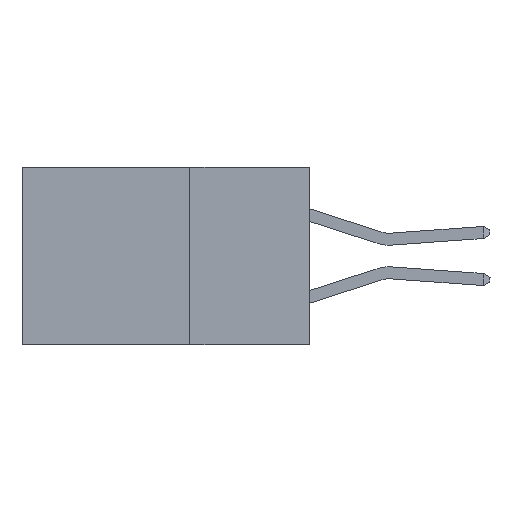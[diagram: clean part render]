
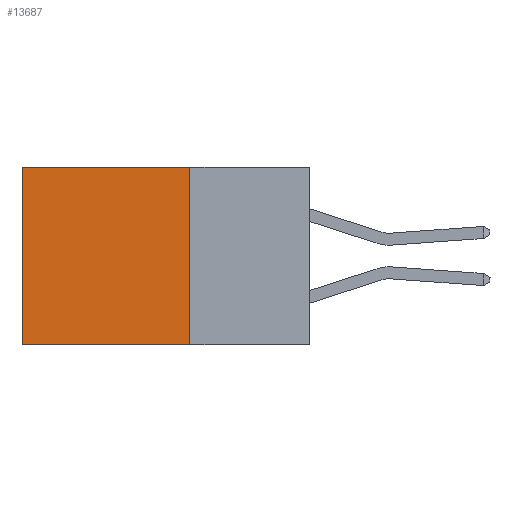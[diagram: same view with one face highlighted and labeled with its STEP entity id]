
A CAD part, left-side view. The second image highlights one B-rep face of the part: STEP entity #13687.
In plain terms, the highlighted planar face has unit normal (-1, 0, 0).
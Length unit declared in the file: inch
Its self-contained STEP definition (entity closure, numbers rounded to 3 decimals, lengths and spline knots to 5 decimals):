
#252 = CARTESIAN_POINT ( 'NONE',  ( 0.2615, 0.25, -0.37 ) ) ;
#585 = LINE ( 'NONE', #252, #17036 ) ;
#797 = CARTESIAN_POINT ( 'NONE',  ( 0.2615, 0.6, -0.37 ) ) ;
#1308 = VERTEX_POINT ( 'NONE', #10513 ) ;
#1394 = DIRECTION ( 'NONE',  ( 0., 0., -1. ) ) ;
#1459 = EDGE_CURVE ( 'NONE', #1308, #5428, #2092, .T. ) ;
#1609 = CARTESIAN_POINT ( 'NONE',  ( 0.2615, 0.6, 0. ) ) ;
#1669 = VERTEX_POINT ( 'NONE', #16102 ) ;
#2092 = LINE ( 'NONE', #4563, #17542 ) ;
#2621 = CARTESIAN_POINT ( 'NONE',  ( 0.2615, 0.25, -0.37 ) ) ;
#2965 = CARTESIAN_POINT ( 'NONE',  ( 0.2615, 0.6, -0.37 ) ) ;
#4163 = DIRECTION ( 'NONE',  ( 0., 0., -1. ) ) ;
#4496 = VECTOR ( 'NONE', #4163, 39.37008 ) ;
#4563 = CARTESIAN_POINT ( 'NONE',  ( 0.2615, 0.25, 0. ) ) ;
#5382 = DIRECTION ( 'NONE',  ( 0., 0., -1. ) ) ;
#5428 = VERTEX_POINT ( 'NONE', #1609 ) ;
#7073 = ORIENTED_EDGE ( 'NONE', *, *, #16119, .F. ) ;
#7903 = VECTOR ( 'NONE', #1394, 39.37008 ) ;
#10006 = PLANE ( 'NONE',  #19805 ) ;
#10513 = CARTESIAN_POINT ( 'NONE',  ( 0.2615, 0.25, 0. ) ) ;
#11168 = DIRECTION ( 'NONE',  ( 0., 1., 0. ) ) ;
#11567 = DIRECTION ( 'NONE',  ( 0., 1., 0. ) ) ;
#12026 = LINE ( 'NONE', #2965, #7903 ) ;
#12293 = LINE ( 'NONE', #2621, #4496 ) ;
#13418 = EDGE_CURVE ( 'NONE', #1308, #1669, #12293, .T. ) ;
#13687 = ADVANCED_FACE ( 'NONE', ( #19135 ), #10006, .F. ) ;
#13839 = ORIENTED_EDGE ( 'NONE', *, *, #16612, .T. ) ;
#14662 = DIRECTION ( 'NONE',  ( 1., 0., 0. ) ) ;
#16102 = CARTESIAN_POINT ( 'NONE',  ( 0.2615, 0.25, -0.37 ) ) ;
#16119 = EDGE_CURVE ( 'NONE', #1669, #19129, #585, .T. ) ;
#16612 = EDGE_CURVE ( 'NONE', #5428, #19129, #12026, .T. ) ;
#17036 = VECTOR ( 'NONE', #11168, 39.37008 ) ;
#17390 = EDGE_LOOP ( 'NONE', ( #13839, #7073, #18435, #18114 ) ) ;
#17542 = VECTOR ( 'NONE', #11567, 39.37008 ) ;
#17615 = CARTESIAN_POINT ( 'NONE',  ( 0.2615, 0.25, -0.37 ) ) ;
#18114 = ORIENTED_EDGE ( 'NONE', *, *, #1459, .T. ) ;
#18435 = ORIENTED_EDGE ( 'NONE', *, *, #13418, .F. ) ;
#19129 = VERTEX_POINT ( 'NONE', #797 ) ;
#19135 = FACE_OUTER_BOUND ( 'NONE', #17390, .T. ) ;
#19805 = AXIS2_PLACEMENT_3D ( 'NONE', #17615, #14662, #5382 ) ;
